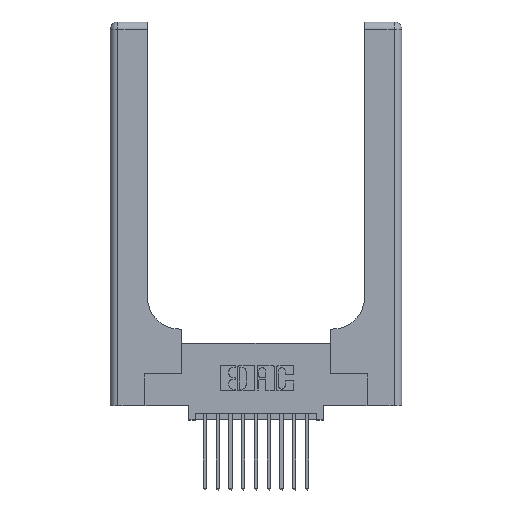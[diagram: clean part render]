
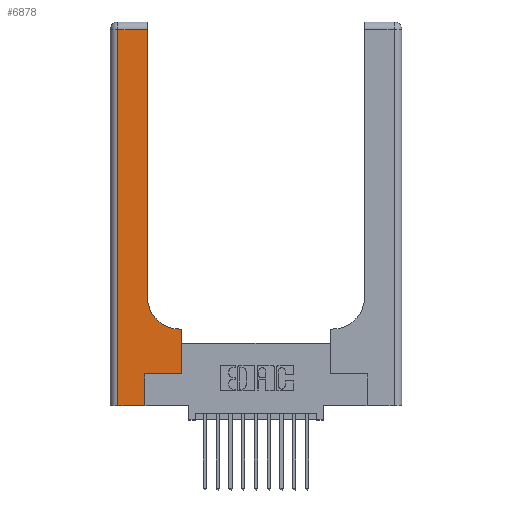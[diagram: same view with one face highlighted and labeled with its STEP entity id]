
A CAD part, top view. The second image highlights one B-rep face of the part: STEP entity #6878.
In plain terms, the highlighted planar face has unit normal (0, 0, 1).
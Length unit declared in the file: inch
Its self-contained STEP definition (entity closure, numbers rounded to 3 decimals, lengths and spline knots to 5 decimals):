
#305 = CARTESIAN_POINT ( 'NONE',  ( 0.5585, 0.25, 0.37 ) ) ;
#448 = DIRECTION ( 'NONE',  ( -1., 0., 0. ) ) ;
#499 = EDGE_CURVE ( 'NONE', #5011, #6667, #11499, .T. ) ;
#667 = CARTESIAN_POINT ( 'NONE',  ( 0.5415, 0.6, 0.37 ) ) ;
#1226 = CARTESIAN_POINT ( 'NONE',  ( 0.06, 0., 0.37 ) ) ;
#1350 = EDGE_CURVE ( 'NONE', #6667, #4888, #3928, .T. ) ;
#1571 = CARTESIAN_POINT ( 'NONE',  ( 0.06, 2.94, 0.37 ) ) ;
#1648 = VERTEX_POINT ( 'NONE', #4995 ) ;
#1755 = CARTESIAN_POINT ( 'NONE',  ( 0., 3., 0.37 ) ) ;
#1908 = LINE ( 'NONE', #16305, #5434 ) ;
#2207 = ORIENTED_EDGE ( 'NONE', *, *, #10981, .T. ) ;
#2219 = CARTESIAN_POINT ( 'NONE',  ( 0.5585, 0.25, 0.37 ) ) ;
#2358 = VECTOR ( 'NONE', #7437, 39.37008 ) ;
#2633 = ORIENTED_EDGE ( 'NONE', *, *, #2676, .T. ) ;
#2676 = EDGE_CURVE ( 'NONE', #3250, #5011, #2836, .T. ) ;
#2836 = LINE ( 'NONE', #12102, #9433 ) ;
#3098 = CARTESIAN_POINT ( 'NONE',  ( 0.5585, 0.6, 0.37 ) ) ;
#3250 = VERTEX_POINT ( 'NONE', #1226 ) ;
#3745 = LINE ( 'NONE', #15862, #10537 ) ;
#3928 = LINE ( 'NONE', #7713, #6613 ) ;
#4888 = VERTEX_POINT ( 'NONE', #305 ) ;
#4995 = CARTESIAN_POINT ( 'NONE',  ( 0.2915, 0.85, 0.37 ) ) ;
#5011 = VERTEX_POINT ( 'NONE', #9831 ) ;
#5353 = CARTESIAN_POINT ( 'NONE',  ( 0.2915, 3., 0.37 ) ) ;
#5434 = VECTOR ( 'NONE', #13746, 39.37008 ) ;
#5500 = CARTESIAN_POINT ( 'NONE',  ( 0.5415, 0.85, 0.37 ) ) ;
#6581 = ORIENTED_EDGE ( 'NONE', *, *, #499, .T. ) ;
#6613 = VECTOR ( 'NONE', #8031, 39.37008 ) ;
#6667 = VERTEX_POINT ( 'NONE', #7325 ) ;
#6670 = VERTEX_POINT ( 'NONE', #667 ) ;
#6816 = EDGE_CURVE ( 'NONE', #8677, #6670, #3745, .T. ) ;
#6849 = DIRECTION ( 'NONE',  ( 1., 0., 0. ) ) ;
#6878 = ADVANCED_FACE ( 'NONE', ( #10144 ), #7108, .F. ) ;
#6907 = LINE ( 'NONE', #2219, #16299 ) ;
#7108 = PLANE ( 'NONE',  #16337 ) ;
#7325 = CARTESIAN_POINT ( 'NONE',  ( 0.269, 0.25, 0.37 ) ) ;
#7355 = VECTOR ( 'NONE', #15649, 39.37008 ) ;
#7406 = ORIENTED_EDGE ( 'NONE', *, *, #6816, .T. ) ;
#7437 = DIRECTION ( 'NONE',  ( -1., 0., 0. ) ) ;
#7713 = CARTESIAN_POINT ( 'NONE',  ( 0.269, 0.25, 0.37 ) ) ;
#8031 = DIRECTION ( 'NONE',  ( 1., 0., 0. ) ) ;
#8090 = VECTOR ( 'NONE', #15770, 39.37008 ) ;
#8451 = DIRECTION ( 'NONE',  ( 0., 0., -1. ) ) ;
#8677 = VERTEX_POINT ( 'NONE', #3098 ) ;
#9433 = VECTOR ( 'NONE', #12040, 39.37008 ) ;
#9541 = EDGE_LOOP ( 'NONE', ( #12231, #2207, #15978, #2633, #6581, #10056, #10455, #7406, #14196 ) ) ;
#9831 = CARTESIAN_POINT ( 'NONE',  ( 0.269, 0., 0.37 ) ) ;
#10056 = ORIENTED_EDGE ( 'NONE', *, *, #1350, .T. ) ;
#10144 = FACE_OUTER_BOUND ( 'NONE', #9541, .T. ) ;
#10443 = VERTEX_POINT ( 'NONE', #11326 ) ;
#10455 = ORIENTED_EDGE ( 'NONE', *, *, #12823, .T. ) ;
#10498 = AXIS2_PLACEMENT_3D ( 'NONE', #5500, #14515, #6849 ) ;
#10537 = VECTOR ( 'NONE', #14649, 39.37008 ) ;
#10981 = EDGE_CURVE ( 'NONE', #10443, #14845, #16135, .T. ) ;
#11326 = CARTESIAN_POINT ( 'NONE',  ( 0.2915, 2.94, 0.37 ) ) ;
#11499 = LINE ( 'NONE', #15732, #8090 ) ;
#11843 = EDGE_CURVE ( 'NONE', #1648, #10443, #14547, .T. ) ;
#12040 = DIRECTION ( 'NONE',  ( 1., 0., 0. ) ) ;
#12102 = CARTESIAN_POINT ( 'NONE',  ( 0., 0., 0.37 ) ) ;
#12231 = ORIENTED_EDGE ( 'NONE', *, *, #11843, .T. ) ;
#12532 = CARTESIAN_POINT ( 'NONE',  ( 0., 2.94, 0.37 ) ) ;
#12663 = DIRECTION ( 'NONE',  ( 0., 1., 0. ) ) ;
#12823 = EDGE_CURVE ( 'NONE', #4888, #8677, #6907, .T. ) ;
#13124 = CIRCLE ( 'NONE', #10498, 0.25 ) ;
#13746 = DIRECTION ( 'NONE',  ( 0., -1., 0. ) ) ;
#14196 = ORIENTED_EDGE ( 'NONE', *, *, #15944, .T. ) ;
#14515 = DIRECTION ( 'NONE',  ( 0., 0., -1. ) ) ;
#14547 = LINE ( 'NONE', #5353, #7355 ) ;
#14649 = DIRECTION ( 'NONE',  ( -1., 0., 0. ) ) ;
#14845 = VERTEX_POINT ( 'NONE', #1571 ) ;
#15521 = EDGE_CURVE ( 'NONE', #14845, #3250, #1908, .T. ) ;
#15649 = DIRECTION ( 'NONE',  ( 0., 1., 0. ) ) ;
#15732 = CARTESIAN_POINT ( 'NONE',  ( 0.269, 0., 0.37 ) ) ;
#15770 = DIRECTION ( 'NONE',  ( 0., 1., 0. ) ) ;
#15862 = CARTESIAN_POINT ( 'NONE',  ( 0.2915, 0.6, 0.37 ) ) ;
#15944 = EDGE_CURVE ( 'NONE', #6670, #1648, #13124, .T. ) ;
#15978 = ORIENTED_EDGE ( 'NONE', *, *, #15521, .T. ) ;
#16135 = LINE ( 'NONE', #12532, #2358 ) ;
#16299 = VECTOR ( 'NONE', #12663, 39.37008 ) ;
#16305 = CARTESIAN_POINT ( 'NONE',  ( 0.06, 3., 0.37 ) ) ;
#16337 = AXIS2_PLACEMENT_3D ( 'NONE', #1755, #8451, #448 ) ;
